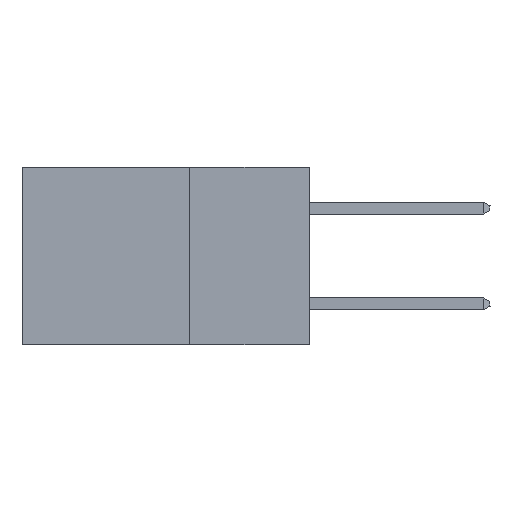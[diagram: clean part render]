
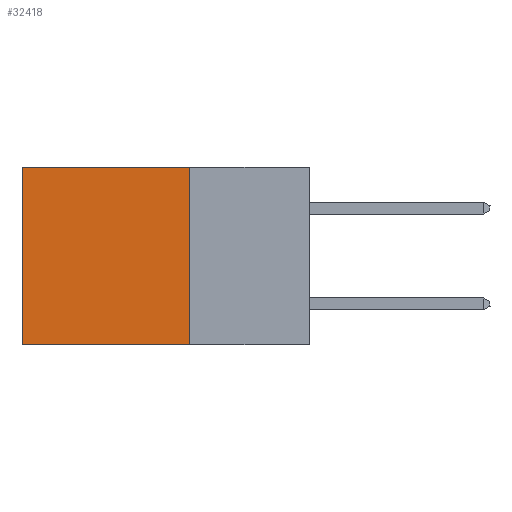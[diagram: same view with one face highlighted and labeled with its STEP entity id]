
A CAD part, left-side view. The second image highlights one B-rep face of the part: STEP entity #32418.
In plain terms, the highlighted planar face has unit normal (-1, 0, 0).
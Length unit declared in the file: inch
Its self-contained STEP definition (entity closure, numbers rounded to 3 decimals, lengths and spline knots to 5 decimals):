
#28 = VERTEX_POINT ( 'NONE', #32404 ) ;
#2028 = DIRECTION ( 'NONE',  ( 0., 0., -1. ) ) ;
#5874 = EDGE_CURVE ( 'NONE', #28343, #14906, #16640, .T. ) ;
#6949 = DIRECTION ( 'NONE',  ( 0., 0., -1. ) ) ;
#7221 = EDGE_CURVE ( 'NONE', #28343, #28, #9649, .T. ) ;
#7273 = CARTESIAN_POINT ( 'NONE',  ( 0.2875, 0.25, 0. ) ) ;
#8720 = PLANE ( 'NONE',  #28938 ) ;
#9196 = EDGE_CURVE ( 'NONE', #14906, #21141, #12806, .T. ) ;
#9649 = LINE ( 'NONE', #22291, #28648 ) ;
#9744 = VECTOR ( 'NONE', #15097, 39.37008 ) ;
#11853 = DIRECTION ( 'NONE',  ( 0., 1., 0. ) ) ;
#12806 = LINE ( 'NONE', #17611, #19700 ) ;
#13917 = DIRECTION ( 'NONE',  ( 1., 0., 0. ) ) ;
#14906 = VERTEX_POINT ( 'NONE', #27913 ) ;
#15097 = DIRECTION ( 'NONE',  ( 0., 1., 0. ) ) ;
#15123 = EDGE_LOOP ( 'NONE', ( #26175, #32529, #17738, #33253 ) ) ;
#16640 = LINE ( 'NONE', #7273, #9744 ) ;
#17611 = CARTESIAN_POINT ( 'NONE',  ( 0.2875, 0.6, 0. ) ) ;
#17738 = ORIENTED_EDGE ( 'NONE', *, *, #7221, .F. ) ;
#18637 = EDGE_CURVE ( 'NONE', #28, #21141, #20681, .T. ) ;
#19467 = FACE_OUTER_BOUND ( 'NONE', #15123, .T. ) ;
#19700 = VECTOR ( 'NONE', #2028, 39.37008 ) ;
#19899 = VECTOR ( 'NONE', #11853, 39.37008 ) ;
#20681 = LINE ( 'NONE', #24724, #19899 ) ;
#21141 = VERTEX_POINT ( 'NONE', #24576 ) ;
#22291 = CARTESIAN_POINT ( 'NONE',  ( 0.2875, 0.25, 0. ) ) ;
#24576 = CARTESIAN_POINT ( 'NONE',  ( 0.2875, 0.6, -0.37 ) ) ;
#24724 = CARTESIAN_POINT ( 'NONE',  ( 0.2875, 0.25, -0.37 ) ) ;
#26175 = ORIENTED_EDGE ( 'NONE', *, *, #9196, .T. ) ;
#26615 = CARTESIAN_POINT ( 'NONE',  ( 0.2875, 0.25, 0. ) ) ;
#27913 = CARTESIAN_POINT ( 'NONE',  ( 0.2875, 0.6, 0. ) ) ;
#28343 = VERTEX_POINT ( 'NONE', #26615 ) ;
#28648 = VECTOR ( 'NONE', #6949, 39.37008 ) ;
#28938 = AXIS2_PLACEMENT_3D ( 'NONE', #29398, #13917, #31989 ) ;
#29398 = CARTESIAN_POINT ( 'NONE',  ( 0.2875, 0.25, 0. ) ) ;
#31989 = DIRECTION ( 'NONE',  ( 0., 0., -1. ) ) ;
#32404 = CARTESIAN_POINT ( 'NONE',  ( 0.2875, 0.25, -0.37 ) ) ;
#32418 = ADVANCED_FACE ( 'NONE', ( #19467 ), #8720, .F. ) ;
#32529 = ORIENTED_EDGE ( 'NONE', *, *, #18637, .F. ) ;
#33253 = ORIENTED_EDGE ( 'NONE', *, *, #5874, .T. ) ;
